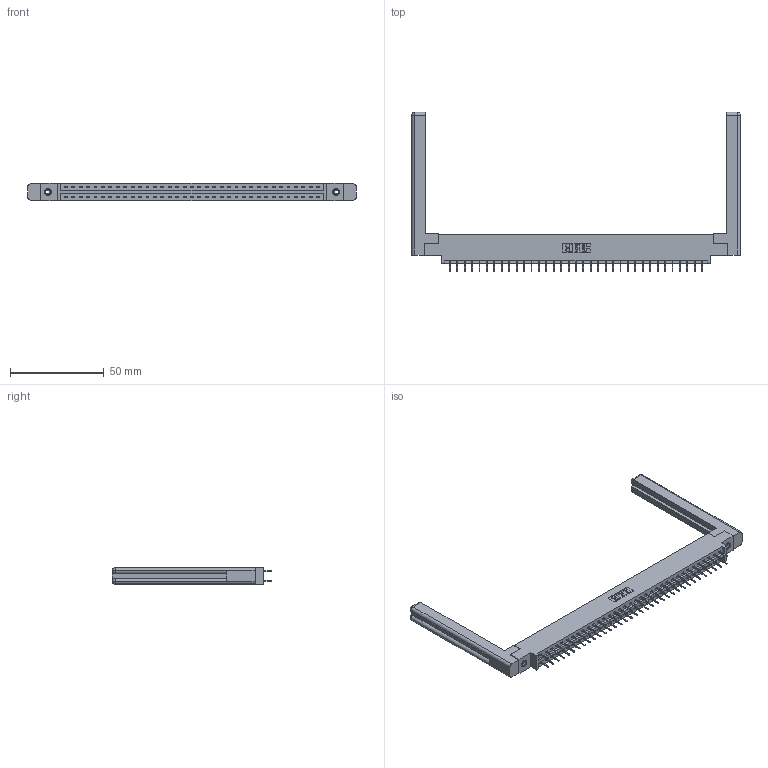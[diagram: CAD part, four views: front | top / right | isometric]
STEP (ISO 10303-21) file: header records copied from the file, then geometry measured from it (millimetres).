
FILE_DESCRIPTION (( 'STEP AP203' ), '1' );
FILE_NAME ('337-070-524-858.STEP', '2019-10-15T10:53:45', ( '' ), ( '' ), 'SwSTEP 2.0', 'SolidWorks 2016', '' );
FILE_SCHEMA (( 'CONFIG_CONTROL_DESIGN' ));
Length unit declared in the file: inch
Products named in the file (5): 337 Part_0.170 Offset - 0.156 Dia-TI; 307-220-058; 345-292-001_345-293-124; 345-250-001_345-250-001-102; 337-070-524-858
Assembly tree (75 placements, depth 2):
  337-070-524-858
    337 Part_0.170 Offset - 0.156 Dia-TI
    345-292-001_345-293-124  x70
    345-250-001_345-250-001-102  x2
    307-220-058  x2
Bounding box: 175.31 x 85.1 x 9.4 mm (x, y, z)
Volume: 25301.4 mm3; surface area: 25287.3 mm2
Topology: 75 solids, 75 shells, 4320 faces, 12227 edges, 7858 vertices
Faces by surface type: plane 3238, cylinder 1058, cone 12, torus 12
Entity records: 30882 total; most frequent: CARTESIAN_POINT 5217, ORIENTED_EDGE 5092, DIRECTION 4466, EDGE_CURVE 2546, VECTOR 2374, LINE 2374, VERTEX_POINT 1686, AXIS2_PLACEMENT_3D 1046
